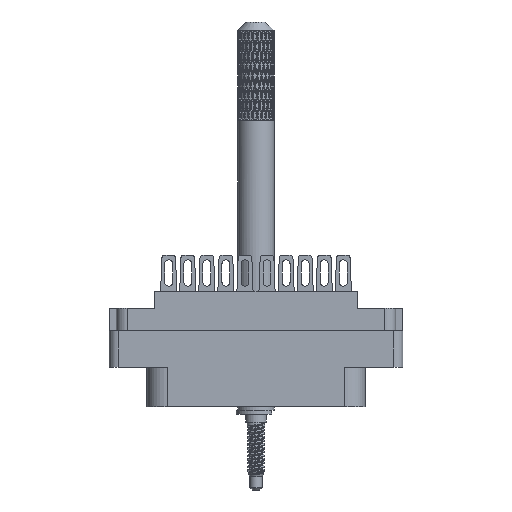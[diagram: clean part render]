
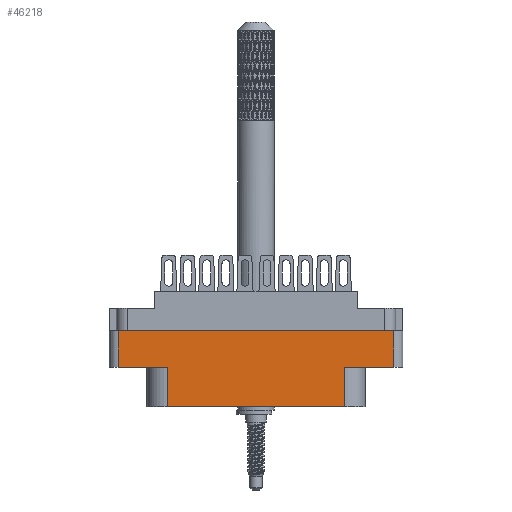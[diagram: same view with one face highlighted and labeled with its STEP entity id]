
A CAD part, front view. The second image highlights one B-rep face of the part: STEP entity #46218.
In plain terms, the highlighted planar face has unit normal (0, -1, 0).
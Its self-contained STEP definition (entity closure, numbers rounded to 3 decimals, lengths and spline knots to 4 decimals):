
#929 = PLANE ( 'NONE',  #50273 ) ;
#1089 = ORIENTED_EDGE ( 'NONE', *, *, #60637, .T. ) ;
#1421 = VERTEX_POINT ( 'NONE', #87660 ) ;
#1588 = ORIENTED_EDGE ( 'NONE', *, *, #20566, .F. ) ;
#3709 = EDGE_CURVE ( 'NONE', #80095, #1421, #83345, .T. ) ;
#3929 = CARTESIAN_POINT ( 'NONE',  ( 0.604, -0.438, -0.52 ) ) ;
#3960 = DIRECTION ( 'NONE',  ( 1., 0., 0. ) ) ;
#3981 = LINE ( 'NONE', #85865, #86526 ) ;
#5806 = ORIENTED_EDGE ( 'NONE', *, *, #3709, .T. ) ;
#7849 = VECTOR ( 'NONE', #60375, 39.3701 ) ;
#8946 = DIRECTION ( 'NONE',  ( 0., -1., 0. ) ) ;
#9661 = CARTESIAN_POINT ( 'NONE',  ( -1., -0.438, -0.789 ) ) ;
#11326 = VERTEX_POINT ( 'NONE', #76265 ) ;
#13544 = DIRECTION ( 'NONE',  ( 1., 0., 0. ) ) ;
#15131 = CARTESIAN_POINT ( 'NONE',  ( -1., -0.438, -0.789 ) ) ;
#16987 = DIRECTION ( 'NONE',  ( 0., 0., -1. ) ) ;
#20403 = EDGE_CURVE ( 'NONE', #11326, #80095, #83108, .T. ) ;
#20566 = EDGE_CURVE ( 'NONE', #36134, #57243, #88057, .T. ) ;
#25244 = VECTOR ( 'NONE', #3960, 39.3701 ) ;
#25731 = EDGE_LOOP ( 'NONE', ( #80189, #102804, #60437, #103369, #5806, #28977, #1588, #1089 ) ) ;
#27146 = CARTESIAN_POINT ( 'NONE',  ( -0.604, -0.438, -0.789 ) ) ;
#27319 = CARTESIAN_POINT ( 'NONE',  ( 0.938, -0.438, -0.52 ) ) ;
#28257 = CARTESIAN_POINT ( 'NONE',  ( -0.604, -0.438, -0.789 ) ) ;
#28977 = ORIENTED_EDGE ( 'NONE', *, *, #88018, .T. ) ;
#33076 = EDGE_CURVE ( 'NONE', #79304, #51552, #96568, .T. ) ;
#33586 = LINE ( 'NONE', #42765, #71146 ) ;
#36134 = VERTEX_POINT ( 'NONE', #27319 ) ;
#41118 = CARTESIAN_POINT ( 'NONE',  ( 0.604, -0.438, -0.52 ) ) ;
#42765 = CARTESIAN_POINT ( 'NONE',  ( 0.938, -0.438, -0.789 ) ) ;
#44138 = DIRECTION ( 'NONE',  ( 0., 0., 1. ) ) ;
#45489 = EDGE_CURVE ( 'NONE', #52523, #11326, #3981, .T. ) ;
#45872 = DIRECTION ( 'NONE',  ( 1., 0., 0. ) ) ;
#46218 = ADVANCED_FACE ( 'NONE', ( #48872 ), #929, .T. ) ;
#48872 = FACE_OUTER_BOUND ( 'NONE', #25731, .T. ) ;
#49129 = LINE ( 'NONE', #3929, #52890 ) ;
#50273 = AXIS2_PLACEMENT_3D ( 'NONE', #9661, #8946, #16987 ) ;
#50338 = LINE ( 'NONE', #99202, #7849 ) ;
#51552 = VERTEX_POINT ( 'NONE', #51841 ) ;
#51841 = CARTESIAN_POINT ( 'NONE',  ( 0.938, -0.438, -0.268 ) ) ;
#52523 = VERTEX_POINT ( 'NONE', #65507 ) ;
#52890 = VECTOR ( 'NONE', #74859, 39.3701 ) ;
#57243 = VERTEX_POINT ( 'NONE', #41118 ) ;
#59253 = VECTOR ( 'NONE', #92267, 39.3701 ) ;
#59509 = CARTESIAN_POINT ( 'NONE',  ( 0., -0.438, -0.268 ) ) ;
#60375 = DIRECTION ( 'NONE',  ( 0., 0., -1. ) ) ;
#60437 = ORIENTED_EDGE ( 'NONE', *, *, #45489, .T. ) ;
#60637 = EDGE_CURVE ( 'NONE', #36134, #51552, #33586, .T. ) ;
#65507 = CARTESIAN_POINT ( 'NONE',  ( -0.938, -0.438, -0.52 ) ) ;
#69301 = VECTOR ( 'NONE', #72104, 39.3701 ) ;
#71146 = VECTOR ( 'NONE', #44138, 39.3701 ) ;
#72104 = DIRECTION ( 'NONE',  ( -1., 0., 0. ) ) ;
#74859 = DIRECTION ( 'NONE',  ( 0., 0., 1. ) ) ;
#76265 = CARTESIAN_POINT ( 'NONE',  ( -0.604, -0.438, -0.52 ) ) ;
#79304 = VERTEX_POINT ( 'NONE', #82965 ) ;
#80095 = VERTEX_POINT ( 'NONE', #27146 ) ;
#80123 = CARTESIAN_POINT ( 'NONE',  ( 0., -0.438, -0.52 ) ) ;
#80189 = ORIENTED_EDGE ( 'NONE', *, *, #33076, .F. ) ;
#82965 = CARTESIAN_POINT ( 'NONE',  ( -0.938, -0.438, -0.268 ) ) ;
#83108 = LINE ( 'NONE', #28257, #59253 ) ;
#83345 = LINE ( 'NONE', #15131, #94527 ) ;
#85865 = CARTESIAN_POINT ( 'NONE',  ( 0., -0.438, -0.52 ) ) ;
#86526 = VECTOR ( 'NONE', #13544, 39.3701 ) ;
#87660 = CARTESIAN_POINT ( 'NONE',  ( 0.604, -0.438, -0.789 ) ) ;
#88018 = EDGE_CURVE ( 'NONE', #1421, #57243, #49129, .T. ) ;
#88057 = LINE ( 'NONE', #80123, #69301 ) ;
#88351 = EDGE_CURVE ( 'NONE', #79304, #52523, #50338, .T. ) ;
#92267 = DIRECTION ( 'NONE',  ( 0., 0., -1. ) ) ;
#94527 = VECTOR ( 'NONE', #45872, 39.3701 ) ;
#96568 = LINE ( 'NONE', #59509, #25244 ) ;
#99202 = CARTESIAN_POINT ( 'NONE',  ( -0.938, -0.438, -0.789 ) ) ;
#102804 = ORIENTED_EDGE ( 'NONE', *, *, #88351, .T. ) ;
#103369 = ORIENTED_EDGE ( 'NONE', *, *, #20403, .T. ) ;
